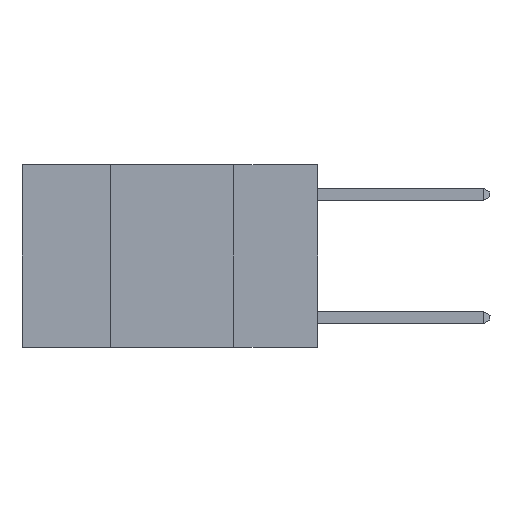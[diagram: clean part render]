
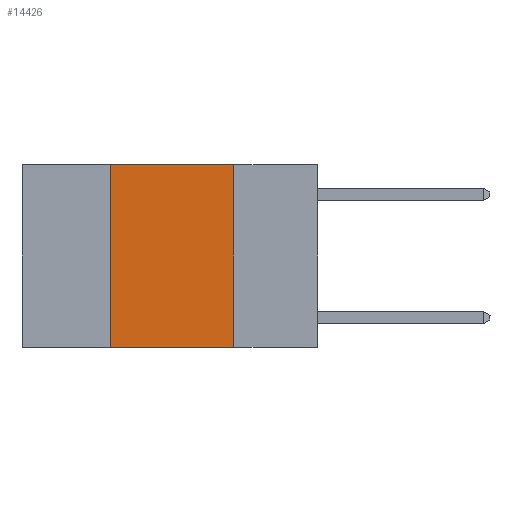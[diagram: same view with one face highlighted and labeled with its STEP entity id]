
A CAD part, left-side view. The second image highlights one B-rep face of the part: STEP entity #14426.
In plain terms, the highlighted planar face has unit normal (-1, 0, 0).
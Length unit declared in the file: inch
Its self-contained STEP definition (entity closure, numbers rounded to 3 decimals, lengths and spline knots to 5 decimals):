
#665 = CARTESIAN_POINT ( 'NONE',  ( 0., 0.17, -0.37 ) ) ;
#1276 = LINE ( 'NONE', #2824, #28072 ) ;
#2725 = VECTOR ( 'NONE', #25125, 39.37008 ) ;
#2824 = CARTESIAN_POINT ( 'NONE',  ( 0., 0.6, 0. ) ) ;
#5875 = CARTESIAN_POINT ( 'NONE',  ( 0., 0.17, 0. ) ) ;
#6057 = LINE ( 'NONE', #5875, #22032 ) ;
#6281 = AXIS2_PLACEMENT_3D ( 'NONE', #13245, #9405, #15415 ) ;
#7067 = ORIENTED_EDGE ( 'NONE', *, *, #15382, .F. ) ;
#8108 = DIRECTION ( 'NONE',  ( 0., 0., -1. ) ) ;
#9004 = EDGE_CURVE ( 'NONE', #27196, #20321, #25820, .T. ) ;
#9405 = DIRECTION ( 'NONE',  ( 1., 0., 0. ) ) ;
#9940 = DIRECTION ( 'NONE',  ( 0., 0., 1. ) ) ;
#11522 = ORIENTED_EDGE ( 'NONE', *, *, #25372, .F. ) ;
#12164 = FACE_OUTER_BOUND ( 'NONE', #24853, .T. ) ;
#12306 = CARTESIAN_POINT ( 'NONE',  ( 0., 0.6, -0.37 ) ) ;
#13245 = CARTESIAN_POINT ( 'NONE',  ( 0., 0.6, 0. ) ) ;
#13747 = CARTESIAN_POINT ( 'NONE',  ( 0., 0.42, -0.37 ) ) ;
#14329 = CARTESIAN_POINT ( 'NONE',  ( 0., 0.42, 0. ) ) ;
#14426 = ADVANCED_FACE ( 'NONE', ( #12164 ), #23934, .F. ) ;
#15382 = EDGE_CURVE ( 'NONE', #26730, #20321, #6057, .T. ) ;
#15415 = DIRECTION ( 'NONE',  ( 0., 0., -1. ) ) ;
#15997 = DIRECTION ( 'NONE',  ( 0., -1., 0. ) ) ;
#17986 = ORIENTED_EDGE ( 'NONE', *, *, #24269, .F. ) ;
#18113 = LINE ( 'NONE', #14329, #23113 ) ;
#18522 = CARTESIAN_POINT ( 'NONE',  ( 0., 0.17, 0. ) ) ;
#19344 = VERTEX_POINT ( 'NONE', #27940 ) ;
#20321 = VERTEX_POINT ( 'NONE', #665 ) ;
#22032 = VECTOR ( 'NONE', #8108, 39.37008 ) ;
#22713 = ORIENTED_EDGE ( 'NONE', *, *, #9004, .T. ) ;
#23113 = VECTOR ( 'NONE', #9940, 39.37008 ) ;
#23934 = PLANE ( 'NONE',  #6281 ) ;
#24269 = EDGE_CURVE ( 'NONE', #19344, #26730, #1276, .T. ) ;
#24853 = EDGE_LOOP ( 'NONE', ( #7067, #17986, #11522, #22713 ) ) ;
#25125 = DIRECTION ( 'NONE',  ( 0., -1., 0. ) ) ;
#25372 = EDGE_CURVE ( 'NONE', #27196, #19344, #18113, .T. ) ;
#25820 = LINE ( 'NONE', #12306, #2725 ) ;
#26730 = VERTEX_POINT ( 'NONE', #18522 ) ;
#27196 = VERTEX_POINT ( 'NONE', #13747 ) ;
#27940 = CARTESIAN_POINT ( 'NONE',  ( 0., 0.42, 0. ) ) ;
#28072 = VECTOR ( 'NONE', #15997, 39.37008 ) ;
